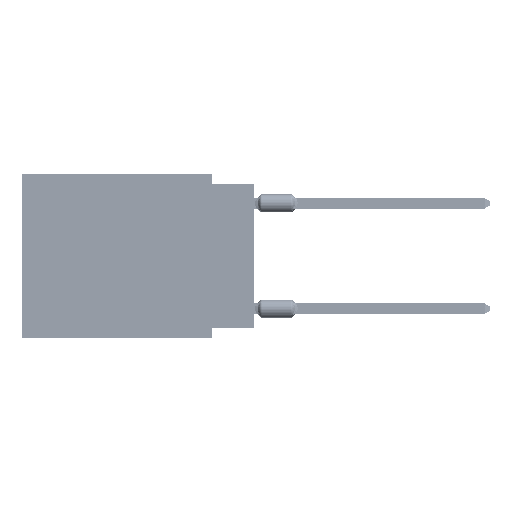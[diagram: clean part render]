
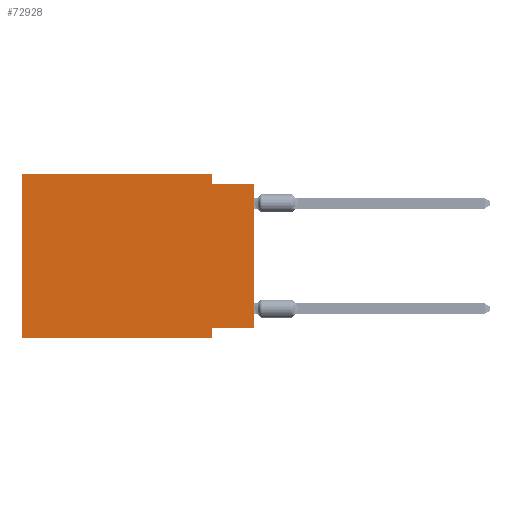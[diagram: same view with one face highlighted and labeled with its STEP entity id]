
A CAD part, left-side view. The second image highlights one B-rep face of the part: STEP entity #72928.
In plain terms, the highlighted planar face has unit normal (-1, 0, 0).
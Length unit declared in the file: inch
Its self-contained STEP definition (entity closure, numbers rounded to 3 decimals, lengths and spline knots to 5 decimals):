
#94 = CARTESIAN_POINT ( 'NONE',  ( 0., 0.55, -0.39 ) ) ;
#178 = VERTEX_POINT ( 'NONE', #48280 ) ;
#840 = LINE ( 'NONE', #46891, #56173 ) ;
#1154 = ORIENTED_EDGE ( 'NONE', *, *, #23094, .F. ) ;
#4269 = CARTESIAN_POINT ( 'NONE',  ( 0., 0.55, 0. ) ) ;
#5023 = VERTEX_POINT ( 'NONE', #94 ) ;
#5374 = VECTOR ( 'NONE', #61291, 39.37008 ) ;
#5398 = CARTESIAN_POINT ( 'NONE',  ( 0., 0.1, -0.365 ) ) ;
#6810 = LINE ( 'NONE', #34392, #53749 ) ;
#8421 = ORIENTED_EDGE ( 'NONE', *, *, #62404, .F. ) ;
#8475 = CARTESIAN_POINT ( 'NONE',  ( 0., 0.55, 0. ) ) ;
#8634 = ORIENTED_EDGE ( 'NONE', *, *, #55118, .T. ) ;
#9500 = ORIENTED_EDGE ( 'NONE', *, *, #11245, .F. ) ;
#10265 = VERTEX_POINT ( 'NONE', #28971 ) ;
#11245 = EDGE_CURVE ( 'NONE', #178, #15333, #13964, .T. ) ;
#12119 = EDGE_CURVE ( 'NONE', #5023, #10265, #60216, .T. ) ;
#13283 = ORIENTED_EDGE ( 'NONE', *, *, #47494, .F. ) ;
#13964 = LINE ( 'NONE', #36975, #71673 ) ;
#14250 = DIRECTION ( 'NONE',  ( 0., 0., 1. ) ) ;
#14293 = AXIS2_PLACEMENT_3D ( 'NONE', #23776, #30182, #48306 ) ;
#15333 = VERTEX_POINT ( 'NONE', #5398 ) ;
#15835 = VECTOR ( 'NONE', #21271, 39.37008 ) ;
#21271 = DIRECTION ( 'NONE',  ( 0., 0., -1. ) ) ;
#21939 = CARTESIAN_POINT ( 'NONE',  ( 0., 0.1, -0.39 ) ) ;
#22998 = VERTEX_POINT ( 'NONE', #21939 ) ;
#23094 = EDGE_CURVE ( 'NONE', #34601, #65017, #6810, .T. ) ;
#23200 = EDGE_CURVE ( 'NONE', #178, #65017, #26300, .T. ) ;
#23776 = CARTESIAN_POINT ( 'NONE',  ( 0., 0.55, 0. ) ) ;
#25643 = ORIENTED_EDGE ( 'NONE', *, *, #12119, .F. ) ;
#26300 = LINE ( 'NONE', #38762, #69422 ) ;
#27835 = ORIENTED_EDGE ( 'NONE', *, *, #23200, .T. ) ;
#28424 = VECTOR ( 'NONE', #63157, 39.37008 ) ;
#28971 = CARTESIAN_POINT ( 'NONE',  ( 0., 0.55, 0. ) ) ;
#30121 = VECTOR ( 'NONE', #66243, 39.37008 ) ;
#30182 = DIRECTION ( 'NONE',  ( 1., 0., 0. ) ) ;
#32084 = CARTESIAN_POINT ( 'NONE',  ( 0., 0.1, -0.025 ) ) ;
#32799 = DIRECTION ( 'NONE',  ( 0., 1., 0. ) ) ;
#34392 = CARTESIAN_POINT ( 'NONE',  ( 0., 0., -0.025 ) ) ;
#34601 = VERTEX_POINT ( 'NONE', #32084 ) ;
#36786 = CARTESIAN_POINT ( 'NONE',  ( 0., 0., -0.025 ) ) ;
#36975 = CARTESIAN_POINT ( 'NONE',  ( 0., 0., -0.365 ) ) ;
#38193 = CARTESIAN_POINT ( 'NONE',  ( 0., 0.1, 0. ) ) ;
#38762 = CARTESIAN_POINT ( 'NONE',  ( 0., 0., 0. ) ) ;
#39360 = LINE ( 'NONE', #4269, #5374 ) ;
#39403 = CARTESIAN_POINT ( 'NONE',  ( 0., 0.1, 0. ) ) ;
#39415 = EDGE_CURVE ( 'NONE', #10265, #41986, #39360, .T. ) ;
#40436 = DIRECTION ( 'NONE',  ( 0., -1., 0. ) ) ;
#41986 = VERTEX_POINT ( 'NONE', #38193 ) ;
#45406 = LINE ( 'NONE', #68433, #28424 ) ;
#46824 = FACE_OUTER_BOUND ( 'NONE', #48468, .T. ) ;
#46891 = CARTESIAN_POINT ( 'NONE',  ( 0., 0.55, -0.39 ) ) ;
#47494 = EDGE_CURVE ( 'NONE', #15333, #22998, #45406, .T. ) ;
#48280 = CARTESIAN_POINT ( 'NONE',  ( 0., 0., -0.365 ) ) ;
#48306 = DIRECTION ( 'NONE',  ( 0., 0., -1. ) ) ;
#48468 = EDGE_LOOP ( 'NONE', ( #27835, #1154, #8421, #52140, #25643, #8634, #13283, #9500 ) ) ;
#51113 = LINE ( 'NONE', #39403, #15835 ) ;
#52140 = ORIENTED_EDGE ( 'NONE', *, *, #39415, .F. ) ;
#53749 = VECTOR ( 'NONE', #40436, 39.37008 ) ;
#55118 = EDGE_CURVE ( 'NONE', #5023, #22998, #840, .T. ) ;
#56173 = VECTOR ( 'NONE', #63172, 39.37008 ) ;
#60216 = LINE ( 'NONE', #8475, #30121 ) ;
#61291 = DIRECTION ( 'NONE',  ( 0., -1., 0. ) ) ;
#62404 = EDGE_CURVE ( 'NONE', #41986, #34601, #51113, .T. ) ;
#63157 = DIRECTION ( 'NONE',  ( 0., 0., -1. ) ) ;
#63172 = DIRECTION ( 'NONE',  ( 0., -1., 0. ) ) ;
#64940 = PLANE ( 'NONE',  #14293 ) ;
#65017 = VERTEX_POINT ( 'NONE', #36786 ) ;
#66243 = DIRECTION ( 'NONE',  ( 0., 0., 1. ) ) ;
#68433 = CARTESIAN_POINT ( 'NONE',  ( 0., 0.1, -0.39 ) ) ;
#69422 = VECTOR ( 'NONE', #14250, 39.37008 ) ;
#71673 = VECTOR ( 'NONE', #32799, 39.37008 ) ;
#72928 = ADVANCED_FACE ( 'NONE', ( #46824 ), #64940, .F. ) ;
